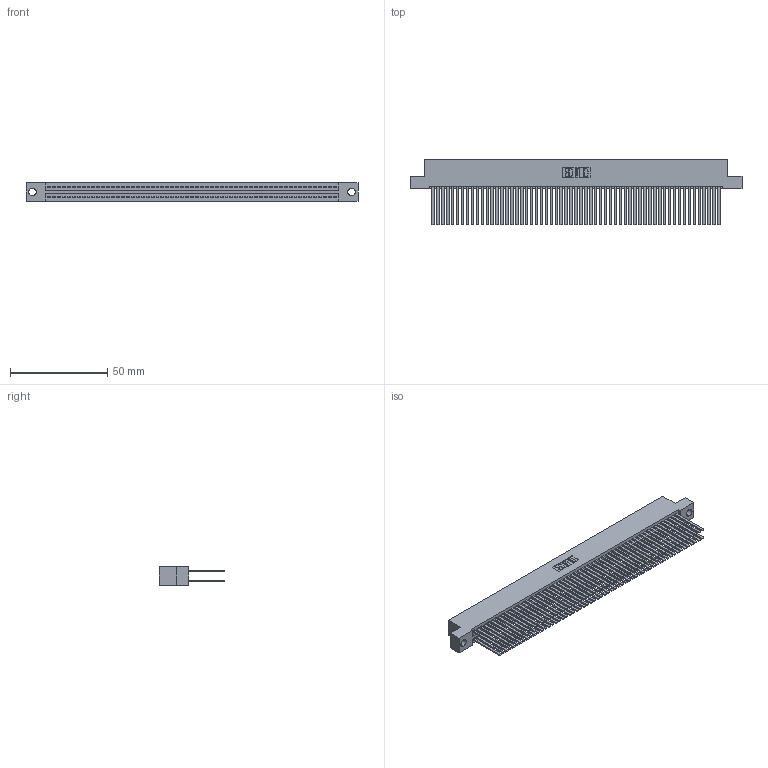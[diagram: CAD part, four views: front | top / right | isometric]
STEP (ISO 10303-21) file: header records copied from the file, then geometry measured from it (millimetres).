
FILE_DESCRIPTION (( 'STEP AP203' ), '1' );
FILE_NAME ('345-118-544-204.STEP', '2021-05-25T16:23:24', ( '' ), ( '' ), 'SwSTEP 2.0', 'SolidWorks 2020', '' );
FILE_SCHEMA (( 'CONFIG_CONTROL_DESIGN' ));
Length unit declared in the file: inch
Products named in the file (3): 345 Part_Flush Mounting Lugs - 0.156 Dia-TI; 345-292-001_345-293-144; 345-118-544-204
Assembly tree (119 placements, depth 2):
  345-118-544-204
    345 Part_Flush Mounting Lugs - 0.156 Dia-TI
    345-292-001_345-293-144  x118
Bounding box: 171.07 x 33.96 x 9.4 mm (x, y, z)
Volume: 18323.8 mm3; surface area: 32114.7 mm2
Topology: 119 solids, 119 shells, 5332 faces, 15835 edges, 10398 vertices
Faces by surface type: plane 3516, cylinder 1816
Entity records: 44239 total; most frequent: CARTESIAN_POINT 7402, ORIENTED_EDGE 7334, DIRECTION 6503, EDGE_CURVE 3667, LINE 3303, VECTOR 3303, VERTEX_POINT 2442, AXIS2_PLACEMENT_3D 1600
